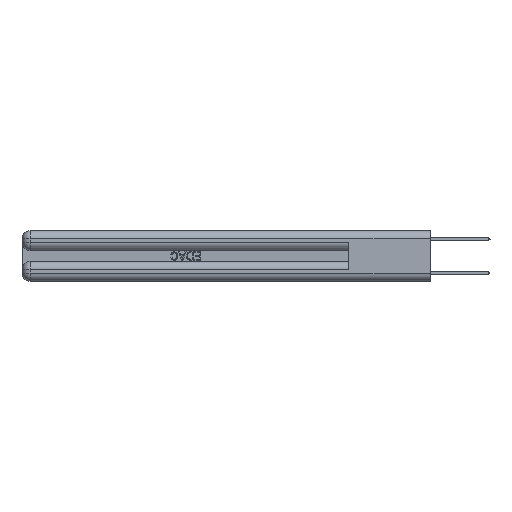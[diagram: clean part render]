
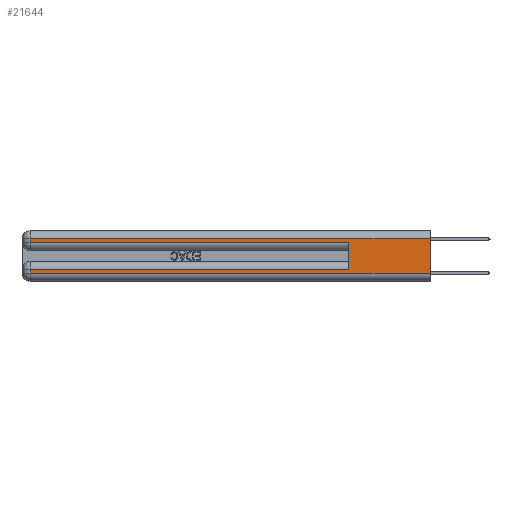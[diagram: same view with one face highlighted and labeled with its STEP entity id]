
A CAD part, left-side view. The second image highlights one B-rep face of the part: STEP entity #21644.
In plain terms, the highlighted planar face has unit normal (-1, 0, 0).
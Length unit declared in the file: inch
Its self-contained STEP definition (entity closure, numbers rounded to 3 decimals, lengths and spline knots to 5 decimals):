
#43 = EDGE_CURVE ( 'NONE', #7114, #17127, #5801, .T. ) ;
#69 = PLANE ( 'NONE',  #28248 ) ;
#801 = LINE ( 'NONE', #14060, #26792 ) ;
#2695 = ORIENTED_EDGE ( 'NONE', *, *, #26686, .F. ) ;
#3210 = EDGE_CURVE ( 'NONE', #13654, #20968, #20387, .T. ) ;
#3732 = VECTOR ( 'NONE', #13951, 39.37008 ) ;
#4346 = LINE ( 'NONE', #26848, #27884 ) ;
#5210 = DIRECTION ( 'NONE',  ( 1., 0., 0. ) ) ;
#5269 = EDGE_CURVE ( 'NONE', #18680, #7114, #18980, .T. ) ;
#5801 = LINE ( 'NONE', #7069, #19625 ) ;
#6056 = CARTESIAN_POINT ( 'NONE',  ( 0., 0.6, 0.285 ) ) ;
#6219 = CARTESIAN_POINT ( 'NONE',  ( 0., 0., 0.06 ) ) ;
#6221 = ORIENTED_EDGE ( 'NONE', *, *, #3210, .T. ) ;
#6763 = DIRECTION ( 'NONE',  ( 0., 0., -1. ) ) ;
#6847 = CARTESIAN_POINT ( 'NONE',  ( 0., 0., 0.31 ) ) ;
#6958 = DIRECTION ( 'NONE',  ( 0., 1., 0. ) ) ;
#7069 = CARTESIAN_POINT ( 'NONE',  ( 0., 0., 0.285 ) ) ;
#7114 = VERTEX_POINT ( 'NONE', #25697 ) ;
#7291 = ORIENTED_EDGE ( 'NONE', *, *, #27436, .F. ) ;
#7871 = CARTESIAN_POINT ( 'NONE',  ( 0., 0., 0.37 ) ) ;
#8179 = DIRECTION ( 'NONE',  ( 0., 0., -1. ) ) ;
#9378 = VECTOR ( 'NONE', #6958, 39.37008 ) ;
#10179 = EDGE_LOOP ( 'NONE', ( #7291, #28372, #21442, #23227, #2695, #6221, #13053, #26433 ) ) ;
#12202 = DIRECTION ( 'NONE',  ( 0., 0., -1. ) ) ;
#12221 = DIRECTION ( 'NONE',  ( 0., 0., -1. ) ) ;
#12520 = CARTESIAN_POINT ( 'NONE',  ( 0., 0.6, 0.085 ) ) ;
#12935 = VECTOR ( 'NONE', #6763, 39.37008 ) ;
#13053 = ORIENTED_EDGE ( 'NONE', *, *, #15978, .T. ) ;
#13296 = CARTESIAN_POINT ( 'NONE',  ( 0., 0., 0.37 ) ) ;
#13654 = VERTEX_POINT ( 'NONE', #12520 ) ;
#13951 = DIRECTION ( 'NONE',  ( 0., 1., 0. ) ) ;
#14060 = CARTESIAN_POINT ( 'NONE',  ( 0., 0., 0.06 ) ) ;
#14707 = VERTEX_POINT ( 'NONE', #29217 ) ;
#14828 = EDGE_CURVE ( 'NONE', #30101, #21967, #801, .T. ) ;
#14850 = FACE_OUTER_BOUND ( 'NONE', #10179, .T. ) ;
#15978 = EDGE_CURVE ( 'NONE', #20968, #30101, #24344, .T. ) ;
#16077 = VECTOR ( 'NONE', #12221, 39.37008 ) ;
#17127 = VERTEX_POINT ( 'NONE', #6056 ) ;
#17845 = VECTOR ( 'NONE', #12202, 39.37008 ) ;
#18680 = VERTEX_POINT ( 'NONE', #31035 ) ;
#18912 = DIRECTION ( 'NONE',  ( 0., 0., 1. ) ) ;
#18980 = LINE ( 'NONE', #20136, #12935 ) ;
#19625 = VECTOR ( 'NONE', #22822, 39.37008 ) ;
#19890 = CARTESIAN_POINT ( 'NONE',  ( 0., 2.94, 0.06 ) ) ;
#20136 = CARTESIAN_POINT ( 'NONE',  ( 0., 2.94, 0.37 ) ) ;
#20387 = LINE ( 'NONE', #22535, #3732 ) ;
#20968 = VERTEX_POINT ( 'NONE', #23416 ) ;
#21442 = ORIENTED_EDGE ( 'NONE', *, *, #5269, .T. ) ;
#21644 = ADVANCED_FACE ( 'NONE', ( #14850 ), #69, .F. ) ;
#21967 = VERTEX_POINT ( 'NONE', #6219 ) ;
#22535 = CARTESIAN_POINT ( 'NONE',  ( 0., 0., 0.085 ) ) ;
#22822 = DIRECTION ( 'NONE',  ( 0., -1., 0. ) ) ;
#23227 = ORIENTED_EDGE ( 'NONE', *, *, #43, .T. ) ;
#23416 = CARTESIAN_POINT ( 'NONE',  ( 0., 2.94, 0.085 ) ) ;
#24019 = EDGE_CURVE ( 'NONE', #14707, #18680, #25203, .T. ) ;
#24344 = LINE ( 'NONE', #25219, #17845 ) ;
#25203 = LINE ( 'NONE', #6847, #9378 ) ;
#25219 = CARTESIAN_POINT ( 'NONE',  ( 0., 2.94, 0.37 ) ) ;
#25697 = CARTESIAN_POINT ( 'NONE',  ( 0., 2.94, 0.285 ) ) ;
#26433 = ORIENTED_EDGE ( 'NONE', *, *, #14828, .T. ) ;
#26686 = EDGE_CURVE ( 'NONE', #13654, #17127, #4346, .T. ) ;
#26792 = VECTOR ( 'NONE', #29667, 39.37008 ) ;
#26848 = CARTESIAN_POINT ( 'NONE',  ( 0., 0.6, 0.145 ) ) ;
#27436 = EDGE_CURVE ( 'NONE', #14707, #21967, #29073, .T. ) ;
#27884 = VECTOR ( 'NONE', #18912, 39.37008 ) ;
#28248 = AXIS2_PLACEMENT_3D ( 'NONE', #13296, #5210, #8179 ) ;
#28372 = ORIENTED_EDGE ( 'NONE', *, *, #24019, .T. ) ;
#29073 = LINE ( 'NONE', #7871, #16077 ) ;
#29217 = CARTESIAN_POINT ( 'NONE',  ( 0., 0., 0.31 ) ) ;
#29667 = DIRECTION ( 'NONE',  ( 0., -1., 0. ) ) ;
#30101 = VERTEX_POINT ( 'NONE', #19890 ) ;
#31035 = CARTESIAN_POINT ( 'NONE',  ( 0., 2.94, 0.31 ) ) ;
